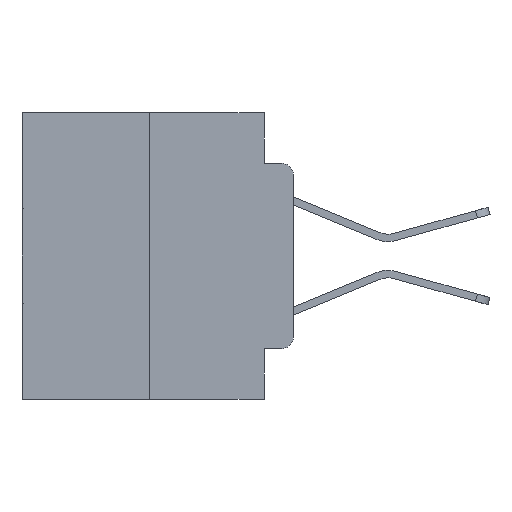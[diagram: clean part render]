
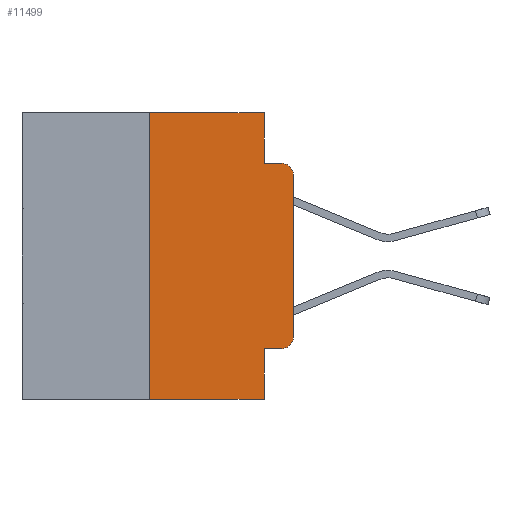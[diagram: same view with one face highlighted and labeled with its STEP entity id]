
A CAD part, left-side view. The second image highlights one B-rep face of the part: STEP entity #11499.
In plain terms, the highlighted planar face has unit normal (-1, 0, 0).
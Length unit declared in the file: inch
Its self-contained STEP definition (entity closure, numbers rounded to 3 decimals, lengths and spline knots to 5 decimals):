
#185 = EDGE_CURVE ( 'NONE', #19396, #23781, #25419, .T. ) ;
#1020 = VERTEX_POINT ( 'NONE', #7005 ) ;
#1763 = EDGE_CURVE ( 'NONE', #1020, #19396, #23348, .T. ) ;
#2162 = DIRECTION ( 'NONE',  ( -1., 0., 0. ) ) ;
#2239 = LINE ( 'NONE', #19740, #13333 ) ;
#2841 = CARTESIAN_POINT ( 'NONE',  ( 0., 0.051, -0.4115 ) ) ;
#3269 = ORIENTED_EDGE ( 'NONE', *, *, #1763, .T. ) ;
#3923 = CIRCLE ( 'NONE', #26024, 0.02 ) ;
#4599 = CARTESIAN_POINT ( 'NONE',  ( 0., 0.473, 0. ) ) ;
#4855 = DIRECTION ( 'NONE',  ( 0., 0., -1. ) ) ;
#5125 = DIRECTION ( 'NONE',  ( 0., -1., 0. ) ) ;
#5320 = VERTEX_POINT ( 'NONE', #27224 ) ;
#5404 = ORIENTED_EDGE ( 'NONE', *, *, #21414, .F. ) ;
#6111 = LINE ( 'NONE', #10499, #22699 ) ;
#6478 = VERTEX_POINT ( 'NONE', #22928 ) ;
#6613 = LINE ( 'NONE', #8196, #16855 ) ;
#6794 = ORIENTED_EDGE ( 'NONE', *, *, #24607, .T. ) ;
#7004 = AXIS2_PLACEMENT_3D ( 'NONE', #9981, #25012, #12151 ) ;
#7005 = CARTESIAN_POINT ( 'NONE',  ( 0., 0., -0.3915 ) ) ;
#7270 = CARTESIAN_POINT ( 'NONE',  ( 0., 0.051, 0. ) ) ;
#7460 = DIRECTION ( 'NONE',  ( 0., -1., 0. ) ) ;
#7781 = VECTOR ( 'NONE', #5125, 39.37008 ) ;
#8171 = ORIENTED_EDGE ( 'NONE', *, *, #15635, .T. ) ;
#8196 = CARTESIAN_POINT ( 'NONE',  ( 0., 0.051, 0. ) ) ;
#8504 = CARTESIAN_POINT ( 'NONE',  ( 0., 0., -0.1085 ) ) ;
#8959 = CARTESIAN_POINT ( 'NONE',  ( 0., 0.02, -0.3915 ) ) ;
#9183 = ORIENTED_EDGE ( 'NONE', *, *, #185, .T. ) ;
#9351 = VECTOR ( 'NONE', #7460, 39.37008 ) ;
#9730 = FACE_OUTER_BOUND ( 'NONE', #23812, .T. ) ;
#9858 = VECTOR ( 'NONE', #24891, 39.37008 ) ;
#9981 = CARTESIAN_POINT ( 'NONE',  ( 0., 0.473, 0. ) ) ;
#10364 = VERTEX_POINT ( 'NONE', #25536 ) ;
#10499 = CARTESIAN_POINT ( 'NONE',  ( 0., 0.051, -0.0885 ) ) ;
#10574 = EDGE_CURVE ( 'NONE', #26379, #24589, #25719, .T. ) ;
#11165 = DIRECTION ( 'NONE',  ( 0., 0., -1. ) ) ;
#11381 = DIRECTION ( 'NONE',  ( 0., 0., 1. ) ) ;
#11499 = ADVANCED_FACE ( 'NONE', ( #9730 ), #22877, .F. ) ;
#11759 = CARTESIAN_POINT ( 'NONE',  ( 0., 0.25, 0. ) ) ;
#12151 = DIRECTION ( 'NONE',  ( 0., 0., -1. ) ) ;
#12658 = DIRECTION ( 'NONE',  ( 0., -1., 0. ) ) ;
#12814 = VERTEX_POINT ( 'NONE', #28198 ) ;
#13333 = VECTOR ( 'NONE', #21909, 39.37008 ) ;
#13654 = VECTOR ( 'NONE', #19836, 39.37008 ) ;
#15635 = EDGE_CURVE ( 'NONE', #5320, #1020, #3923, .T. ) ;
#16855 = VECTOR ( 'NONE', #23399, 39.37008 ) ;
#17111 = EDGE_CURVE ( 'NONE', #10364, #5320, #19302, .T. ) ;
#18828 = CARTESIAN_POINT ( 'NONE',  ( 0., 0.25, -0.5 ) ) ;
#19022 = ORIENTED_EDGE ( 'NONE', *, *, #19956, .F. ) ;
#19302 = LINE ( 'NONE', #2841, #7781 ) ;
#19396 = VERTEX_POINT ( 'NONE', #8504 ) ;
#19504 = LINE ( 'NONE', #20441, #9351 ) ;
#19638 = CARTESIAN_POINT ( 'NONE',  ( 0., 0.02, -0.0885 ) ) ;
#19740 = CARTESIAN_POINT ( 'NONE',  ( 0., 0.25, 0. ) ) ;
#19836 = DIRECTION ( 'NONE',  ( 0., -1., 0. ) ) ;
#19873 = VERTEX_POINT ( 'NONE', #18828 ) ;
#19956 = EDGE_CURVE ( 'NONE', #10364, #12814, #6613, .T. ) ;
#20441 = CARTESIAN_POINT ( 'NONE',  ( 0., 0.473, -0.5 ) ) ;
#21377 = ORIENTED_EDGE ( 'NONE', *, *, #27087, .F. ) ;
#21414 = EDGE_CURVE ( 'NONE', #19873, #26379, #2239, .T. ) ;
#21884 = CARTESIAN_POINT ( 'NONE',  ( 0., 0., 0. ) ) ;
#21909 = DIRECTION ( 'NONE',  ( 0., 0., 1. ) ) ;
#22038 = ORIENTED_EDGE ( 'NONE', *, *, #10574, .F. ) ;
#22068 = AXIS2_PLACEMENT_3D ( 'NONE', #22078, #2162, #4855 ) ;
#22078 = CARTESIAN_POINT ( 'NONE',  ( 0., 0.02, -0.1085 ) ) ;
#22670 = VECTOR ( 'NONE', #11381, 39.37008 ) ;
#22699 = VECTOR ( 'NONE', #12658, 39.37008 ) ;
#22752 = CARTESIAN_POINT ( 'NONE',  ( 0., 0.051, 0. ) ) ;
#22815 = EDGE_CURVE ( 'NONE', #24589, #6478, #26980, .T. ) ;
#22877 = PLANE ( 'NONE',  #7004 ) ;
#22928 = CARTESIAN_POINT ( 'NONE',  ( 0., 0.051, -0.0885 ) ) ;
#23348 = LINE ( 'NONE', #21884, #22670 ) ;
#23399 = DIRECTION ( 'NONE',  ( 0., 0., -1. ) ) ;
#23781 = VERTEX_POINT ( 'NONE', #19638 ) ;
#23812 = EDGE_LOOP ( 'NONE', ( #3269, #9183, #21377, #27007, #22038, #5404, #6794, #19022, #24684, #8171 ) ) ;
#24056 = DIRECTION ( 'NONE',  ( -1., 0., 0. ) ) ;
#24589 = VERTEX_POINT ( 'NONE', #7270 ) ;
#24607 = EDGE_CURVE ( 'NONE', #19873, #12814, #19504, .T. ) ;
#24684 = ORIENTED_EDGE ( 'NONE', *, *, #17111, .T. ) ;
#24891 = DIRECTION ( 'NONE',  ( 0., 0., -1. ) ) ;
#25012 = DIRECTION ( 'NONE',  ( 1., 0., 0. ) ) ;
#25419 = CIRCLE ( 'NONE', #22068, 0.02 ) ;
#25536 = CARTESIAN_POINT ( 'NONE',  ( 0., 0.051, -0.4115 ) ) ;
#25719 = LINE ( 'NONE', #4599, #13654 ) ;
#26024 = AXIS2_PLACEMENT_3D ( 'NONE', #8959, #24056, #11165 ) ;
#26379 = VERTEX_POINT ( 'NONE', #11759 ) ;
#26980 = LINE ( 'NONE', #22752, #9858 ) ;
#27007 = ORIENTED_EDGE ( 'NONE', *, *, #22815, .F. ) ;
#27087 = EDGE_CURVE ( 'NONE', #6478, #23781, #6111, .T. ) ;
#27224 = CARTESIAN_POINT ( 'NONE',  ( 0., 0.02, -0.4115 ) ) ;
#28198 = CARTESIAN_POINT ( 'NONE',  ( 0., 0.051, -0.5 ) ) ;
